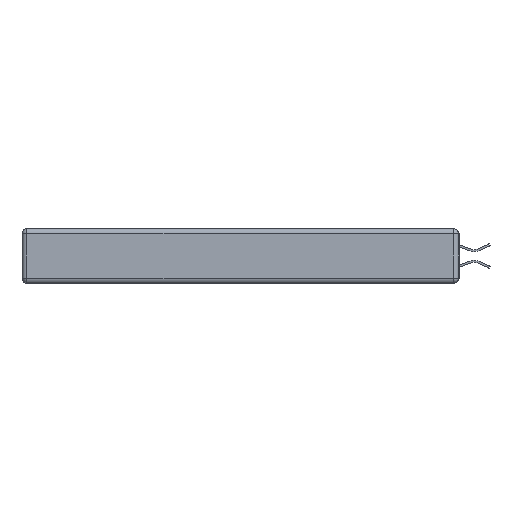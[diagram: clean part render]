
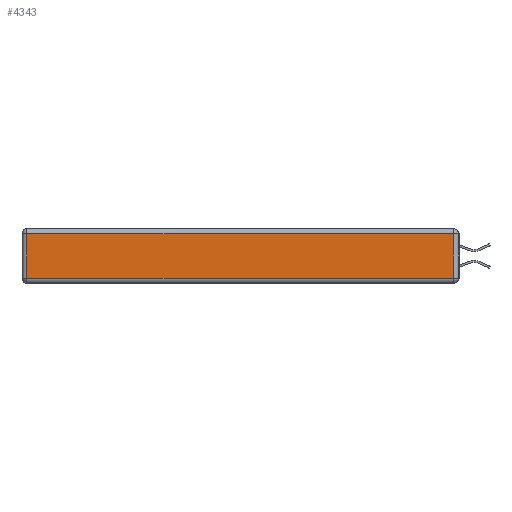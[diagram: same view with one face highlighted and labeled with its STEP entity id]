
A CAD part, left-side view. The second image highlights one B-rep face of the part: STEP entity #4343.
In plain terms, the highlighted planar face has unit normal (-1, 0, 0).
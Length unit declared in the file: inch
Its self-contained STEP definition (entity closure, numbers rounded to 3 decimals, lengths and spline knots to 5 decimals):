
#55 = DIRECTION ( 'NONE',  ( -1., 0., 0. ) ) ;
#331 = ORIENTED_EDGE ( 'NONE', *, *, #12470, .T. ) ;
#595 = DIRECTION ( 'NONE',  ( 0., 0., 1. ) ) ;
#700 = VECTOR ( 'NONE', #595, 39.37008 ) ;
#814 = DIRECTION ( 'NONE',  ( 0., 0., -1. ) ) ;
#1470 = EDGE_CURVE ( 'NONE', #4683, #5213, #17721, .T. ) ;
#1513 = LINE ( 'NONE', #9508, #6047 ) ;
#1856 = VECTOR ( 'NONE', #18170, 39.37008 ) ;
#2976 = VECTOR ( 'NONE', #814, 39.37008 ) ;
#3449 = CARTESIAN_POINT ( 'NONE',  ( 0., 2.72, -0.313 ) ) ;
#3913 = FACE_OUTER_BOUND ( 'NONE', #6244, .T. ) ;
#4343 = ADVANCED_FACE ( 'NONE', ( #3913 ), #15898, .T. ) ;
#4532 = VERTEX_POINT ( 'NONE', #4591 ) ;
#4591 = CARTESIAN_POINT ( 'NONE',  ( 0., 0.03, -0.313 ) ) ;
#4683 = VERTEX_POINT ( 'NONE', #15731 ) ;
#4952 = CARTESIAN_POINT ( 'NONE',  ( 0., 0.03, -0.343 ) ) ;
#5213 = VERTEX_POINT ( 'NONE', #15418 ) ;
#5219 = DIRECTION ( 'NONE',  ( 0., -1., 0. ) ) ;
#5659 = CARTESIAN_POINT ( 'NONE',  ( 0., 0., -0.343 ) ) ;
#6047 = VECTOR ( 'NONE', #5219, 39.37008 ) ;
#6244 = EDGE_LOOP ( 'NONE', ( #14151, #14122, #17942, #331 ) ) ;
#6469 = CARTESIAN_POINT ( 'NONE',  ( 0., 2.72, -0.343 ) ) ;
#7246 = LINE ( 'NONE', #6469, #2976 ) ;
#7450 = EDGE_CURVE ( 'NONE', #14925, #4532, #1513, .T. ) ;
#8011 = CARTESIAN_POINT ( 'NONE',  ( 0., 2.75, -0.03 ) ) ;
#9508 = CARTESIAN_POINT ( 'NONE',  ( 0., 0., -0.313 ) ) ;
#10149 = DIRECTION ( 'NONE',  ( 0., 0., 1. ) ) ;
#12470 = EDGE_CURVE ( 'NONE', #5213, #14925, #7246, .T. ) ;
#12911 = LINE ( 'NONE', #4952, #700 ) ;
#13215 = AXIS2_PLACEMENT_3D ( 'NONE', #5659, #55, #10149 ) ;
#14122 = ORIENTED_EDGE ( 'NONE', *, *, #16073, .T. ) ;
#14151 = ORIENTED_EDGE ( 'NONE', *, *, #7450, .T. ) ;
#14925 = VERTEX_POINT ( 'NONE', #3449 ) ;
#15418 = CARTESIAN_POINT ( 'NONE',  ( 0., 2.72, -0.03 ) ) ;
#15731 = CARTESIAN_POINT ( 'NONE',  ( 0., 0.03, -0.03 ) ) ;
#15898 = PLANE ( 'NONE',  #13215 ) ;
#16073 = EDGE_CURVE ( 'NONE', #4532, #4683, #12911, .T. ) ;
#17721 = LINE ( 'NONE', #8011, #1856 ) ;
#17942 = ORIENTED_EDGE ( 'NONE', *, *, #1470, .T. ) ;
#18170 = DIRECTION ( 'NONE',  ( 0., 1., 0. ) ) ;
